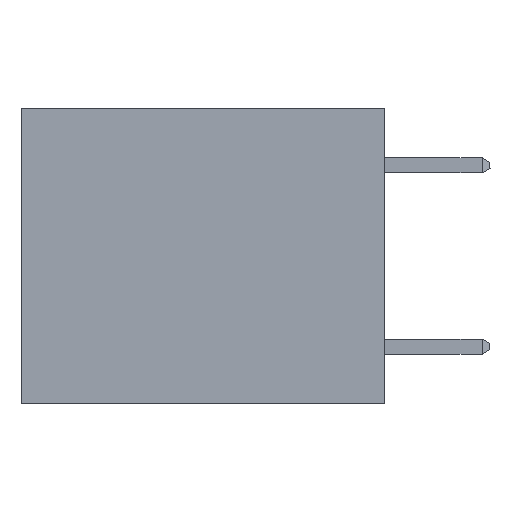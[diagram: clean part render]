
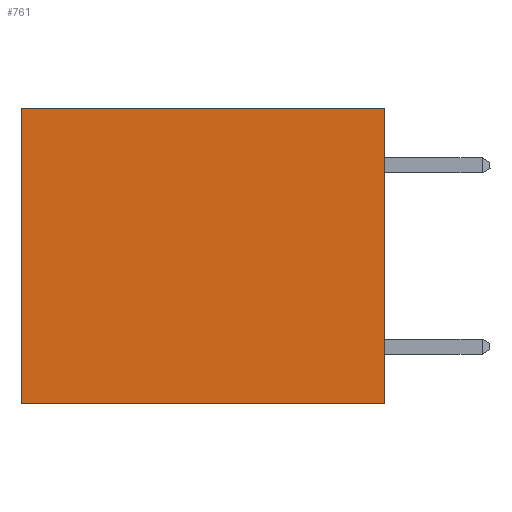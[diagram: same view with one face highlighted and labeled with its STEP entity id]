
A CAD part, left-side view. The second image highlights one B-rep face of the part: STEP entity #761.
In plain terms, the highlighted planar face has unit normal (-1, 0, 0).
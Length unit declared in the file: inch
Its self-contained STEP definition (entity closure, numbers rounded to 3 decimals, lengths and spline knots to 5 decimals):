
#592 = DIRECTION ( 'NONE',  ( 0., 0., -1. ) ) ;
#657 = LINE ( 'NONE', #17127, #22615 ) ;
#719 = AXIS2_PLACEMENT_3D ( 'NONE', #12240, #12079, #23188 ) ;
#761 = ADVANCED_FACE ( 'NONE', ( #22548 ), #19676, .F. ) ;
#1390 = CARTESIAN_POINT ( 'NONE',  ( 0.3165, 0., -0.49 ) ) ;
#2504 = VERTEX_POINT ( 'NONE', #1390 ) ;
#2534 = LINE ( 'NONE', #5645, #16868 ) ;
#4432 = EDGE_CURVE ( 'NONE', #13459, #20162, #6589, .T. ) ;
#5645 = CARTESIAN_POINT ( 'NONE',  ( 0.3165, 0., 0. ) ) ;
#6104 = DIRECTION ( 'NONE',  ( 0., 0., -1. ) ) ;
#6589 = LINE ( 'NONE', #10218, #22980 ) ;
#7278 = CARTESIAN_POINT ( 'NONE',  ( 0.3165, 0., 0. ) ) ;
#7770 = EDGE_CURVE ( 'NONE', #20001, #2504, #657, .T. ) ;
#8679 = ORIENTED_EDGE ( 'NONE', *, *, #4432, .T. ) ;
#9985 = ORIENTED_EDGE ( 'NONE', *, *, #20380, .T. ) ;
#10218 = CARTESIAN_POINT ( 'NONE',  ( 0.3165, 0.6, -0.49 ) ) ;
#11835 = CARTESIAN_POINT ( 'NONE',  ( 0.3165, 0., -0.49 ) ) ;
#12079 = DIRECTION ( 'NONE',  ( 1., 0., 0. ) ) ;
#12240 = CARTESIAN_POINT ( 'NONE',  ( 0.3165, 0., -0.49 ) ) ;
#12511 = ORIENTED_EDGE ( 'NONE', *, *, #23539, .F. ) ;
#13027 = CARTESIAN_POINT ( 'NONE',  ( 0.3165, 0.6, 0. ) ) ;
#13459 = VERTEX_POINT ( 'NONE', #13027 ) ;
#13675 = EDGE_LOOP ( 'NONE', ( #8679, #12511, #13891, #9985 ) ) ;
#13891 = ORIENTED_EDGE ( 'NONE', *, *, #7770, .F. ) ;
#16868 = VECTOR ( 'NONE', #18933, 39.37008 ) ;
#17127 = CARTESIAN_POINT ( 'NONE',  ( 0.3165, 0., -0.49 ) ) ;
#17586 = LINE ( 'NONE', #11835, #20508 ) ;
#17773 = CARTESIAN_POINT ( 'NONE',  ( 0.3165, 0.6, -0.49 ) ) ;
#18933 = DIRECTION ( 'NONE',  ( 0., 1., 0. ) ) ;
#19676 = PLANE ( 'NONE',  #719 ) ;
#20001 = VERTEX_POINT ( 'NONE', #7278 ) ;
#20162 = VERTEX_POINT ( 'NONE', #17773 ) ;
#20380 = EDGE_CURVE ( 'NONE', #20001, #13459, #2534, .T. ) ;
#20508 = VECTOR ( 'NONE', #22944, 39.37008 ) ;
#22548 = FACE_OUTER_BOUND ( 'NONE', #13675, .T. ) ;
#22615 = VECTOR ( 'NONE', #6104, 39.37008 ) ;
#22944 = DIRECTION ( 'NONE',  ( 0., 1., 0. ) ) ;
#22980 = VECTOR ( 'NONE', #592, 39.37008 ) ;
#23188 = DIRECTION ( 'NONE',  ( 0., 0., -1. ) ) ;
#23539 = EDGE_CURVE ( 'NONE', #2504, #20162, #17586, .T. ) ;
